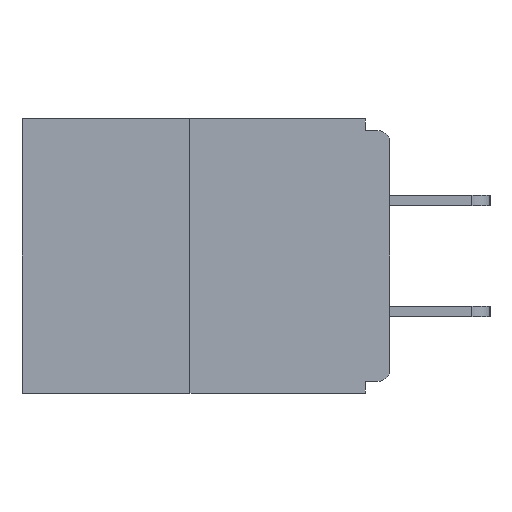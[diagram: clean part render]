
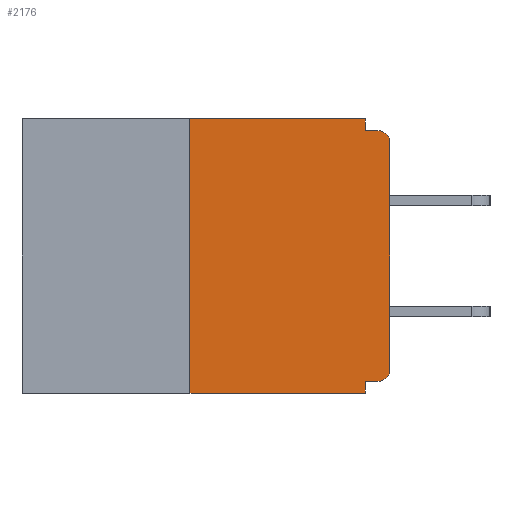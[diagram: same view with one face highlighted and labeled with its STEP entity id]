
A CAD part, left-side view. The second image highlights one B-rep face of the part: STEP entity #2176.
In plain terms, the highlighted planar face has unit normal (-1, 0, 0).
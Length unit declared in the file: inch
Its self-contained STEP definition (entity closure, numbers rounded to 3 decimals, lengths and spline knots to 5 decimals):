
#24 = VERTEX_POINT ( 'NONE', #13013 ) ;
#137 = CARTESIAN_POINT ( 'NONE',  ( 0., 0., 0. ) ) ;
#1037 = ORIENTED_EDGE ( 'NONE', *, *, #12954, .F. ) ;
#1094 = DIRECTION ( 'NONE',  ( 0., 0., -1. ) ) ;
#1238 = CARTESIAN_POINT ( 'NONE',  ( 0., 0.46, -0.343 ) ) ;
#1317 = CARTESIAN_POINT ( 'NONE',  ( 0., 0.25, 0. ) ) ;
#1947 = LINE ( 'NONE', #3515, #14072 ) ;
#2176 = ADVANCED_FACE ( 'NONE', ( #5680 ), #20338, .F. ) ;
#2442 = EDGE_CURVE ( 'NONE', #24, #16045, #7663, .T. ) ;
#2772 = EDGE_CURVE ( 'NONE', #4585, #8593, #2815, .T. ) ;
#2815 = LINE ( 'NONE', #1238, #11371 ) ;
#2836 = DIRECTION ( 'NONE',  ( 0., 1., 0. ) ) ;
#3053 = DIRECTION ( 'NONE',  ( 0., 0., 1. ) ) ;
#3066 = CARTESIAN_POINT ( 'NONE',  ( 0., 0.031, -0.328 ) ) ;
#3515 = CARTESIAN_POINT ( 'NONE',  ( 0., 0.25, 0. ) ) ;
#3554 = EDGE_CURVE ( 'NONE', #12229, #6352, #9899, .T. ) ;
#3688 = CARTESIAN_POINT ( 'NONE',  ( 0., 0., -0.313 ) ) ;
#3724 = VERTEX_POINT ( 'NONE', #3688 ) ;
#3750 = CARTESIAN_POINT ( 'NONE',  ( 0., 0.015, -0.015 ) ) ;
#4110 = CARTESIAN_POINT ( 'NONE',  ( 0., 0.46, 0. ) ) ;
#4215 = VERTEX_POINT ( 'NONE', #16933 ) ;
#4585 = VERTEX_POINT ( 'NONE', #13239 ) ;
#5227 = ORIENTED_EDGE ( 'NONE', *, *, #11144, .F. ) ;
#5680 = FACE_OUTER_BOUND ( 'NONE', #14908, .T. ) ;
#6300 = AXIS2_PLACEMENT_3D ( 'NONE', #8874, #15297, #1094 ) ;
#6352 = VERTEX_POINT ( 'NONE', #3750 ) ;
#6690 = DIRECTION ( 'NONE',  ( 0., 0., -1. ) ) ;
#6900 = CARTESIAN_POINT ( 'NONE',  ( 0., 0.031, 0. ) ) ;
#6999 = LINE ( 'NONE', #6900, #7684 ) ;
#7663 = LINE ( 'NONE', #14097, #8718 ) ;
#7684 = VECTOR ( 'NONE', #6690, 39.37008 ) ;
#8059 = ORIENTED_EDGE ( 'NONE', *, *, #9576, .T. ) ;
#8141 = ORIENTED_EDGE ( 'NONE', *, *, #3554, .T. ) ;
#8313 = EDGE_CURVE ( 'NONE', #15613, #10262, #19001, .T. ) ;
#8330 = CARTESIAN_POINT ( 'NONE',  ( 0., 0., -0.03 ) ) ;
#8593 = VERTEX_POINT ( 'NONE', #19866 ) ;
#8718 = VECTOR ( 'NONE', #2836, 39.37008 ) ;
#8874 = CARTESIAN_POINT ( 'NONE',  ( 0., 0.015, -0.313 ) ) ;
#9576 = EDGE_CURVE ( 'NONE', #24, #3724, #17400, .T. ) ;
#9899 = CIRCLE ( 'NONE', #16953, 0.015 ) ;
#9909 = VECTOR ( 'NONE', #10595, 39.37008 ) ;
#10262 = VERTEX_POINT ( 'NONE', #16303 ) ;
#10539 = DIRECTION ( 'NONE',  ( 0., 0., -1. ) ) ;
#10595 = DIRECTION ( 'NONE',  ( 0., -1., 0. ) ) ;
#10817 = DIRECTION ( 'NONE',  ( 0., -1., 0. ) ) ;
#11080 = AXIS2_PLACEMENT_3D ( 'NONE', #4110, #20237, #10539 ) ;
#11144 = EDGE_CURVE ( 'NONE', #16045, #8593, #13087, .T. ) ;
#11199 = DIRECTION ( 'NONE',  ( 0., 0., -1. ) ) ;
#11260 = LINE ( 'NONE', #137, #13135 ) ;
#11371 = VECTOR ( 'NONE', #10817, 39.37008 ) ;
#11396 = EDGE_CURVE ( 'NONE', #4585, #15613, #1947, .T. ) ;
#11793 = VECTOR ( 'NONE', #19914, 39.37008 ) ;
#12015 = ORIENTED_EDGE ( 'NONE', *, *, #14042, .F. ) ;
#12229 = VERTEX_POINT ( 'NONE', #8330 ) ;
#12954 = EDGE_CURVE ( 'NONE', #10262, #4215, #6999, .T. ) ;
#13013 = CARTESIAN_POINT ( 'NONE',  ( 0., 0.015, -0.328 ) ) ;
#13087 = LINE ( 'NONE', #19507, #16452 ) ;
#13135 = VECTOR ( 'NONE', #3053, 39.37008 ) ;
#13239 = CARTESIAN_POINT ( 'NONE',  ( 0., 0.25, -0.343 ) ) ;
#13481 = CARTESIAN_POINT ( 'NONE',  ( 0., 0., -0.015 ) ) ;
#13569 = ORIENTED_EDGE ( 'NONE', *, *, #2772, .T. ) ;
#13959 = EDGE_CURVE ( 'NONE', #3724, #12229, #11260, .T. ) ;
#14042 = EDGE_CURVE ( 'NONE', #4215, #6352, #16543, .T. ) ;
#14072 = VECTOR ( 'NONE', #19535, 39.37008 ) ;
#14097 = CARTESIAN_POINT ( 'NONE',  ( 0., 0., -0.328 ) ) ;
#14554 = DIRECTION ( 'NONE',  ( 0., 0., -1. ) ) ;
#14908 = EDGE_LOOP ( 'NONE', ( #15551, #19202, #13569, #5227, #19663, #8059, #19318, #8141, #12015, #1037 ) ) ;
#15297 = DIRECTION ( 'NONE',  ( -1., 0., 0. ) ) ;
#15551 = ORIENTED_EDGE ( 'NONE', *, *, #8313, .F. ) ;
#15613 = VERTEX_POINT ( 'NONE', #1317 ) ;
#16045 = VERTEX_POINT ( 'NONE', #3066 ) ;
#16303 = CARTESIAN_POINT ( 'NONE',  ( 0., 0.031, 0. ) ) ;
#16452 = VECTOR ( 'NONE', #14554, 39.37008 ) ;
#16543 = LINE ( 'NONE', #13481, #11793 ) ;
#16933 = CARTESIAN_POINT ( 'NONE',  ( 0., 0.031, -0.015 ) ) ;
#16953 = AXIS2_PLACEMENT_3D ( 'NONE', #19305, #17414, #11199 ) ;
#17400 = CIRCLE ( 'NONE', #6300, 0.015 ) ;
#17414 = DIRECTION ( 'NONE',  ( -1., 0., 0. ) ) ;
#18912 = CARTESIAN_POINT ( 'NONE',  ( 0., 0.46, 0. ) ) ;
#19001 = LINE ( 'NONE', #18912, #9909 ) ;
#19202 = ORIENTED_EDGE ( 'NONE', *, *, #11396, .F. ) ;
#19305 = CARTESIAN_POINT ( 'NONE',  ( 0., 0.015, -0.03 ) ) ;
#19318 = ORIENTED_EDGE ( 'NONE', *, *, #13959, .T. ) ;
#19507 = CARTESIAN_POINT ( 'NONE',  ( 0., 0.031, -0.343 ) ) ;
#19535 = DIRECTION ( 'NONE',  ( 0., 0., 1. ) ) ;
#19663 = ORIENTED_EDGE ( 'NONE', *, *, #2442, .F. ) ;
#19866 = CARTESIAN_POINT ( 'NONE',  ( 0., 0.031, -0.343 ) ) ;
#19914 = DIRECTION ( 'NONE',  ( 0., -1., 0. ) ) ;
#20237 = DIRECTION ( 'NONE',  ( 1., 0., 0. ) ) ;
#20338 = PLANE ( 'NONE',  #11080 ) ;
